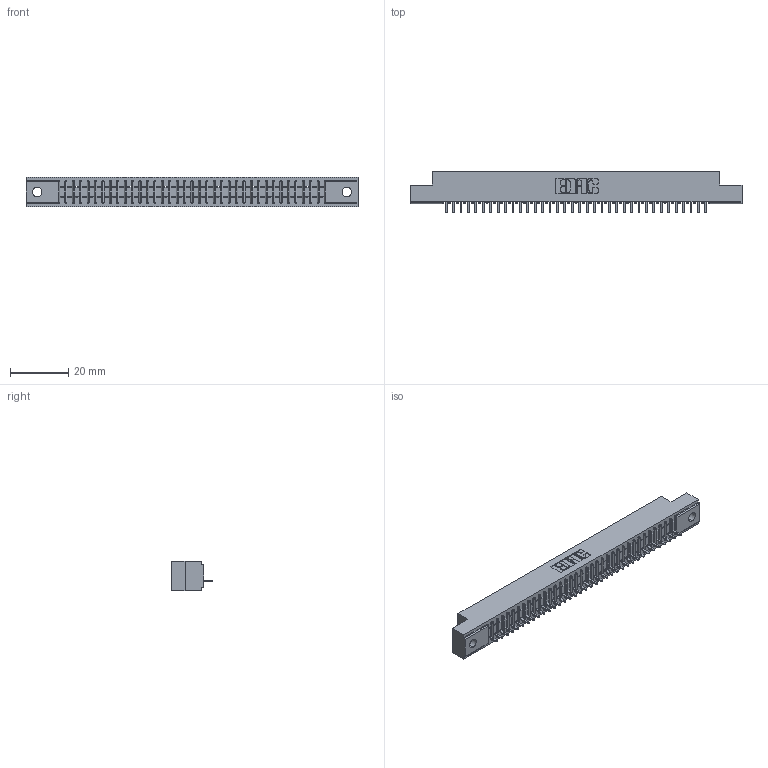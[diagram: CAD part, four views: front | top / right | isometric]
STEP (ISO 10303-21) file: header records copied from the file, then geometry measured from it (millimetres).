
FILE_DESCRIPTION (( 'STEP AP203' ), '1' );
FILE_NAME ('341-036-520-102.STEP', '2018-08-06T22:22:20', ( '' ), ( '' ), 'SwSTEP 2.0', 'SolidWorks 2016', '' );
FILE_SCHEMA (( 'CONFIG_CONTROL_DESIGN' ));
Length unit declared in the file: inch
Products named in the file (3): 341-036-520-102; 341 Part_.128 (3.25) Dia Mounting Holes; 341-292-001_341-292-120
Assembly tree (37 placements, depth 2):
  341-036-520-102
    341 Part_.128 (3.25) Dia Mounting Holes
    341-292-001_341-292-120  x36
Bounding box: 113.67 x 14.27 x 10.16 mm (x, y, z)
Volume: 8091.9 mm3; surface area: 12097.5 mm2
Topology: 37 solids, 37 shells, 3068 faces, 8848 edges, 5678 vertices
Faces by surface type: plane 1904, cylinder 1020, sphere 74, torus 70
Entity records: 43217 total; most frequent: CARTESIAN_POINT 7340, ORIENTED_EDGE 7328, DIRECTION 7090, EDGE_CURVE 3664, LINE 2954, VECTOR 2954, VERTEX_POINT 2318, AXIS2_PLACEMENT_3D 2068
